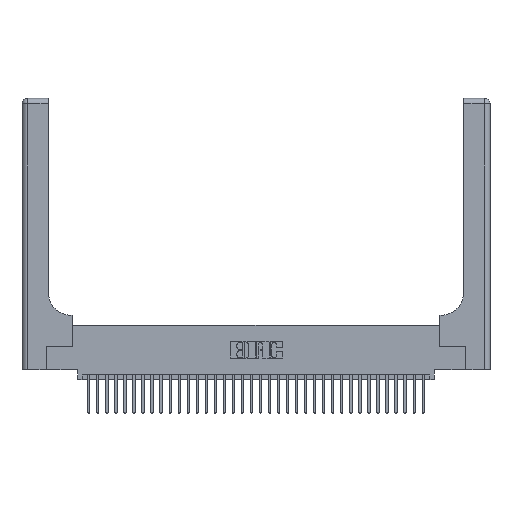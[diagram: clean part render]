
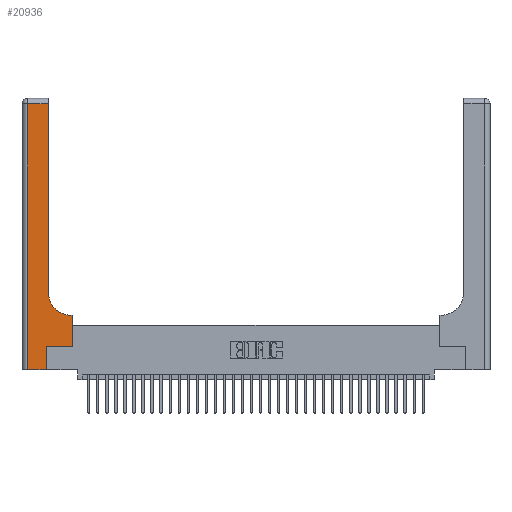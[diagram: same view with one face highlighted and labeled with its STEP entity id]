
A CAD part, top view. The second image highlights one B-rep face of the part: STEP entity #20936.
In plain terms, the highlighted planar face has unit normal (0, 0, 1).
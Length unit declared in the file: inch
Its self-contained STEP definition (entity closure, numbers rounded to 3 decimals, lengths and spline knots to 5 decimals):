
#368 = VECTOR ( 'NONE', #6695, 39.37008 ) ;
#859 = ORIENTED_EDGE ( 'NONE', *, *, #7268, .T. ) ;
#1052 = CARTESIAN_POINT ( 'NONE',  ( 0.269, 0., 0.37 ) ) ;
#1337 = CARTESIAN_POINT ( 'NONE',  ( 0.2915, 0.85, 0.37 ) ) ;
#1964 = CARTESIAN_POINT ( 'NONE',  ( 0.2915, 0.6, 0.37 ) ) ;
#2385 = EDGE_CURVE ( 'NONE', #5008, #27027, #14721, .T. ) ;
#3051 = LINE ( 'NONE', #14660, #24249 ) ;
#3825 = DIRECTION ( 'NONE',  ( 0., 1., 0. ) ) ;
#3920 = CARTESIAN_POINT ( 'NONE',  ( 0.06, 3., 0.37 ) ) ;
#5008 = VERTEX_POINT ( 'NONE', #35481 ) ;
#5386 = CARTESIAN_POINT ( 'NONE',  ( 0.5585, 0.25, 0.37 ) ) ;
#5816 = CARTESIAN_POINT ( 'NONE',  ( 0., 3., 0.37 ) ) ;
#5976 = EDGE_LOOP ( 'NONE', ( #859, #6900, #25111, #26815, #6083, #30681, #17761, #12126, #23011 ) ) ;
#6083 = ORIENTED_EDGE ( 'NONE', *, *, #32530, .T. ) ;
#6185 = CARTESIAN_POINT ( 'NONE',  ( 0.5415, 0.85, 0.37 ) ) ;
#6376 = AXIS2_PLACEMENT_3D ( 'NONE', #6185, #25530, #8951 ) ;
#6666 = DIRECTION ( 'NONE',  ( 0., 1., 0. ) ) ;
#6695 = DIRECTION ( 'NONE',  ( 0., -1., 0. ) ) ;
#6900 = ORIENTED_EDGE ( 'NONE', *, *, #10451, .T. ) ;
#6978 = VERTEX_POINT ( 'NONE', #1337 ) ;
#7268 = EDGE_CURVE ( 'NONE', #6978, #26753, #31262, .T. ) ;
#7681 = LINE ( 'NONE', #3920, #368 ) ;
#8060 = CARTESIAN_POINT ( 'NONE',  ( 0.2915, 3., 0.37 ) ) ;
#8316 = VERTEX_POINT ( 'NONE', #27471 ) ;
#8584 = DIRECTION ( 'NONE',  ( 0., 0., -1. ) ) ;
#8826 = EDGE_CURVE ( 'NONE', #26680, #8316, #30715, .T. ) ;
#8951 = DIRECTION ( 'NONE',  ( 1., 0., 0. ) ) ;
#9416 = CIRCLE ( 'NONE', #6376, 0.25 ) ;
#9938 = LINE ( 'NONE', #17656, #29366 ) ;
#10237 = CARTESIAN_POINT ( 'NONE',  ( 0.269, 0., 0.37 ) ) ;
#10451 = EDGE_CURVE ( 'NONE', #26753, #33552, #3051, .T. ) ;
#10937 = DIRECTION ( 'NONE',  ( 1., 0., 0. ) ) ;
#11977 = DIRECTION ( 'NONE',  ( -1., 0., 0. ) ) ;
#12126 = ORIENTED_EDGE ( 'NONE', *, *, #8826, .T. ) ;
#13050 = CARTESIAN_POINT ( 'NONE',  ( 0.06, 0., 0.37 ) ) ;
#13415 = FACE_OUTER_BOUND ( 'NONE', #5976, .T. ) ;
#14060 = EDGE_CURVE ( 'NONE', #28118, #23764, #30729, .T. ) ;
#14660 = CARTESIAN_POINT ( 'NONE',  ( 0., 2.94, 0.37 ) ) ;
#14721 = LINE ( 'NONE', #30122, #28546 ) ;
#16444 = EDGE_CURVE ( 'NONE', #8316, #6978, #9416, .T. ) ;
#17226 = CARTESIAN_POINT ( 'NONE',  ( 0., 0., 0.37 ) ) ;
#17656 = CARTESIAN_POINT ( 'NONE',  ( 0.5585, 0.25, 0.37 ) ) ;
#17761 = ORIENTED_EDGE ( 'NONE', *, *, #26105, .T. ) ;
#17852 = CARTESIAN_POINT ( 'NONE',  ( 0.5585, 0.6, 0.37 ) ) ;
#18474 = VECTOR ( 'NONE', #3825, 39.37008 ) ;
#19677 = AXIS2_PLACEMENT_3D ( 'NONE', #5816, #8584, #27919 ) ;
#19839 = CARTESIAN_POINT ( 'NONE',  ( 0.06, 2.94, 0.37 ) ) ;
#20936 = ADVANCED_FACE ( 'NONE', ( #13415 ), #22404, .F. ) ;
#22404 = PLANE ( 'NONE',  #19677 ) ;
#23011 = ORIENTED_EDGE ( 'NONE', *, *, #16444, .T. ) ;
#23445 = VECTOR ( 'NONE', #29582, 39.37008 ) ;
#23462 = VECTOR ( 'NONE', #33700, 39.37008 ) ;
#23764 = VERTEX_POINT ( 'NONE', #10237 ) ;
#24249 = VECTOR ( 'NONE', #11977, 39.37008 ) ;
#24670 = DIRECTION ( 'NONE',  ( 0., 1., 0. ) ) ;
#25111 = ORIENTED_EDGE ( 'NONE', *, *, #27348, .T. ) ;
#25530 = DIRECTION ( 'NONE',  ( 0., 0., -1. ) ) ;
#26105 = EDGE_CURVE ( 'NONE', #27027, #26680, #9938, .T. ) ;
#26680 = VERTEX_POINT ( 'NONE', #17852 ) ;
#26695 = LINE ( 'NONE', #1052, #18474 ) ;
#26753 = VERTEX_POINT ( 'NONE', #29174 ) ;
#26815 = ORIENTED_EDGE ( 'NONE', *, *, #14060, .T. ) ;
#27027 = VERTEX_POINT ( 'NONE', #5386 ) ;
#27348 = EDGE_CURVE ( 'NONE', #33552, #28118, #7681, .T. ) ;
#27471 = CARTESIAN_POINT ( 'NONE',  ( 0.5415, 0.6, 0.37 ) ) ;
#27919 = DIRECTION ( 'NONE',  ( -1., 0., 0. ) ) ;
#28118 = VERTEX_POINT ( 'NONE', #13050 ) ;
#28546 = VECTOR ( 'NONE', #10937, 39.37008 ) ;
#28701 = VECTOR ( 'NONE', #24670, 39.37008 ) ;
#29174 = CARTESIAN_POINT ( 'NONE',  ( 0.2915, 2.94, 0.37 ) ) ;
#29366 = VECTOR ( 'NONE', #6666, 39.37008 ) ;
#29582 = DIRECTION ( 'NONE',  ( -1., 0., 0. ) ) ;
#30122 = CARTESIAN_POINT ( 'NONE',  ( 0.269, 0.25, 0.37 ) ) ;
#30681 = ORIENTED_EDGE ( 'NONE', *, *, #2385, .T. ) ;
#30715 = LINE ( 'NONE', #1964, #23445 ) ;
#30729 = LINE ( 'NONE', #17226, #23462 ) ;
#31262 = LINE ( 'NONE', #8060, #28701 ) ;
#32530 = EDGE_CURVE ( 'NONE', #23764, #5008, #26695, .T. ) ;
#33552 = VERTEX_POINT ( 'NONE', #19839 ) ;
#33700 = DIRECTION ( 'NONE',  ( 1., 0., 0. ) ) ;
#35481 = CARTESIAN_POINT ( 'NONE',  ( 0.269, 0.25, 0.37 ) ) ;
